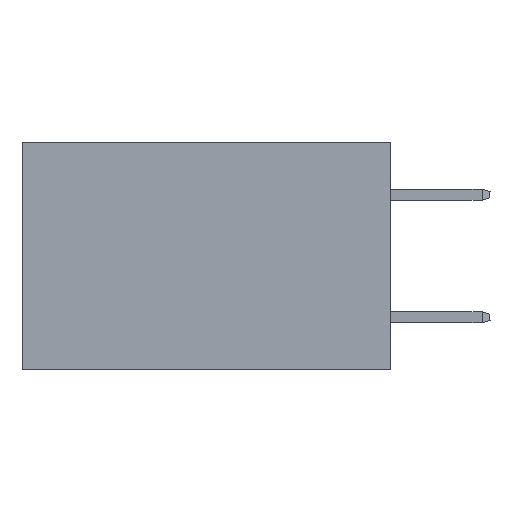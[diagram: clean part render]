
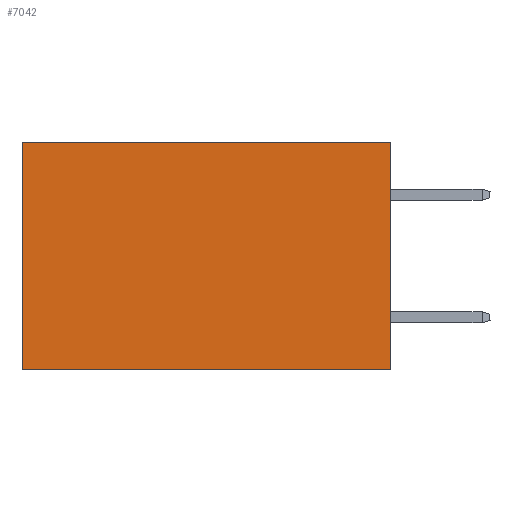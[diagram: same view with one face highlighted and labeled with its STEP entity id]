
A CAD part, left-side view. The second image highlights one B-rep face of the part: STEP entity #7042.
In plain terms, the highlighted planar face has unit normal (-1, 0, 0).
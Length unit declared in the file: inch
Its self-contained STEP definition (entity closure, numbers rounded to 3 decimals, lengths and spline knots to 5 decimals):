
#203 = CARTESIAN_POINT ( 'NONE',  ( 0.2875, 0.6, 0. ) ) ;
#444 = DIRECTION ( 'NONE',  ( 0., 0., -1. ) ) ;
#1460 = AXIS2_PLACEMENT_3D ( 'NONE', #5314, #7292, #444 ) ;
#1492 = VECTOR ( 'NONE', #10028, 39.37008 ) ;
#1507 = DIRECTION ( 'NONE',  ( 0., 0., -1. ) ) ;
#1594 = CARTESIAN_POINT ( 'NONE',  ( 0.2875, 0., 0. ) ) ;
#1895 = VERTEX_POINT ( 'NONE', #9353 ) ;
#2168 = CARTESIAN_POINT ( 'NONE',  ( 0.2875, 0.6, -0.37 ) ) ;
#2316 = PLANE ( 'NONE',  #1460 ) ;
#2703 = EDGE_CURVE ( 'NONE', #1895, #3753, #8823, .T. ) ;
#3209 = VECTOR ( 'NONE', #4019, 39.37008 ) ;
#3542 = CARTESIAN_POINT ( 'NONE',  ( 0.2875, 0., -0.37 ) ) ;
#3713 = FACE_OUTER_BOUND ( 'NONE', #6847, .T. ) ;
#3753 = VERTEX_POINT ( 'NONE', #2168 ) ;
#4019 = DIRECTION ( 'NONE',  ( 0., 1., 0. ) ) ;
#4348 = ORIENTED_EDGE ( 'NONE', *, *, #8889, .F. ) ;
#5239 = ORIENTED_EDGE ( 'NONE', *, *, #11302, .F. ) ;
#5314 = CARTESIAN_POINT ( 'NONE',  ( 0.2875, 0., 0. ) ) ;
#6033 = DIRECTION ( 'NONE',  ( 0., 1., 0. ) ) ;
#6340 = LINE ( 'NONE', #1594, #11804 ) ;
#6847 = EDGE_LOOP ( 'NONE', ( #7197, #4348, #5239, #10914 ) ) ;
#7042 = ADVANCED_FACE ( 'NONE', ( #3713 ), #2316, .F. ) ;
#7197 = ORIENTED_EDGE ( 'NONE', *, *, #2703, .T. ) ;
#7292 = DIRECTION ( 'NONE',  ( 1., 0., 0. ) ) ;
#8823 = LINE ( 'NONE', #203, #1492 ) ;
#8889 = EDGE_CURVE ( 'NONE', #11441, #3753, #11686, .T. ) ;
#9353 = CARTESIAN_POINT ( 'NONE',  ( 0.2875, 0.6, 0. ) ) ;
#9577 = CARTESIAN_POINT ( 'NONE',  ( 0.2875, 0., 0. ) ) ;
#9647 = VECTOR ( 'NONE', #6033, 39.37008 ) ;
#9804 = CARTESIAN_POINT ( 'NONE',  ( 0.2875, 0., 0. ) ) ;
#10028 = DIRECTION ( 'NONE',  ( 0., 0., -1. ) ) ;
#10914 = ORIENTED_EDGE ( 'NONE', *, *, #12173, .T. ) ;
#11302 = EDGE_CURVE ( 'NONE', #12358, #11441, #6340, .T. ) ;
#11441 = VERTEX_POINT ( 'NONE', #3542 ) ;
#11686 = LINE ( 'NONE', #11723, #3209 ) ;
#11723 = CARTESIAN_POINT ( 'NONE',  ( 0.2875, 0., -0.37 ) ) ;
#11804 = VECTOR ( 'NONE', #1507, 39.37008 ) ;
#12173 = EDGE_CURVE ( 'NONE', #12358, #1895, #12223, .T. ) ;
#12223 = LINE ( 'NONE', #9804, #9647 ) ;
#12358 = VERTEX_POINT ( 'NONE', #9577 ) ;
